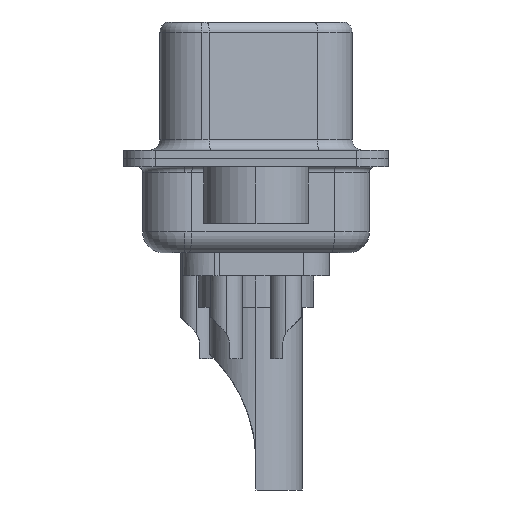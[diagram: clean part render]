
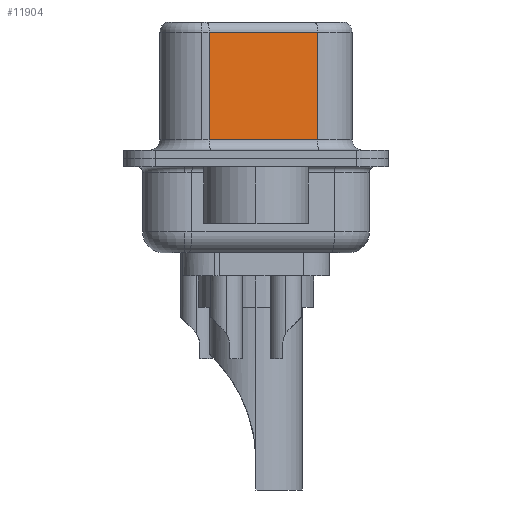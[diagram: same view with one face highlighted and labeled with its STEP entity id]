
A CAD part, left-side view. The second image highlights one B-rep face of the part: STEP entity #11904.
In plain terms, the highlighted planar face has unit normal (-0.985, -0.174, 0).
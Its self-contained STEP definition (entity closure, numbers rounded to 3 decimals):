
#238 = FACE_OUTER_BOUND ( 'NONE', #21168, .T. ) ;
#552 = PLANE ( 'NONE',  #8166 ) ;
#665 = CARTESIAN_POINT ( 'NONE',  ( 4.585, -2.927, 6.52 ) ) ;
#1724 = ORIENTED_EDGE ( 'NONE', *, *, #5225, .T. ) ;
#2642 = VECTOR ( 'NONE', #15337, 1000. ) ;
#3847 = EDGE_CURVE ( 'NONE', #14947, #14819, #8509, .T. ) ;
#3955 = CARTESIAN_POINT ( 'NONE',  ( 3.675, 2.233, 0.9 ) ) ;
#4397 = ORIENTED_EDGE ( 'NONE', *, *, #9425, .F. ) ;
#4581 = EDGE_CURVE ( 'NONE', #12418, #22338, #9320, .T. ) ;
#4880 = CARTESIAN_POINT ( 'NONE',  ( 3.675, 2.233, 6.02 ) ) ;
#5225 = EDGE_CURVE ( 'NONE', #14819, #12418, #17825, .T. ) ;
#5715 = ORIENTED_EDGE ( 'NONE', *, *, #3847, .T. ) ;
#5811 = LINE ( 'NONE', #665, #2642 ) ;
#6054 = DIRECTION ( 'NONE',  ( 0.985, 0.174, 0. ) ) ;
#7430 = CARTESIAN_POINT ( 'NONE',  ( 3.675, 2.233, 6.52 ) ) ;
#7813 = CARTESIAN_POINT ( 'NONE',  ( 4.585, -2.927, 6.52 ) ) ;
#8166 = AXIS2_PLACEMENT_3D ( 'NONE', #7813, #6054, #22595 ) ;
#8509 = LINE ( 'NONE', #13000, #15047 ) ;
#9273 = DIRECTION ( 'NONE',  ( 0., 0., -1. ) ) ;
#9320 = LINE ( 'NONE', #9773, #17013 ) ;
#9425 = EDGE_CURVE ( 'NONE', #14947, #22338, #5811, .T. ) ;
#9773 = CARTESIAN_POINT ( 'NONE',  ( 4.585, -2.927, 0.9 ) ) ;
#11904 = ADVANCED_FACE ( 'NONE', ( #238 ), #552, .F. ) ;
#12418 = VERTEX_POINT ( 'NONE', #3955 ) ;
#13000 = CARTESIAN_POINT ( 'NONE',  ( 4.585, -2.927, 6.02 ) ) ;
#13014 = VECTOR ( 'NONE', #9273, 1000. ) ;
#13625 = CARTESIAN_POINT ( 'NONE',  ( 4.585, -2.927, 6.02 ) ) ;
#13859 = ORIENTED_EDGE ( 'NONE', *, *, #4581, .T. ) ;
#14819 = VERTEX_POINT ( 'NONE', #4880 ) ;
#14947 = VERTEX_POINT ( 'NONE', #13625 ) ;
#15047 = VECTOR ( 'NONE', #20431, 1000. ) ;
#15337 = DIRECTION ( 'NONE',  ( 0., 0., -1. ) ) ;
#17013 = VECTOR ( 'NONE', #23129, 1000. ) ;
#17825 = LINE ( 'NONE', #7430, #13014 ) ;
#17862 = CARTESIAN_POINT ( 'NONE',  ( 4.585, -2.927, 0.9 ) ) ;
#20431 = DIRECTION ( 'NONE',  ( -0.174, 0.985, 0. ) ) ;
#21168 = EDGE_LOOP ( 'NONE', ( #4397, #5715, #1724, #13859 ) ) ;
#22338 = VERTEX_POINT ( 'NONE', #17862 ) ;
#22595 = DIRECTION ( 'NONE',  ( -0.174, 0.985, 0. ) ) ;
#23129 = DIRECTION ( 'NONE',  ( 0.174, -0.985, 0. ) ) ;
